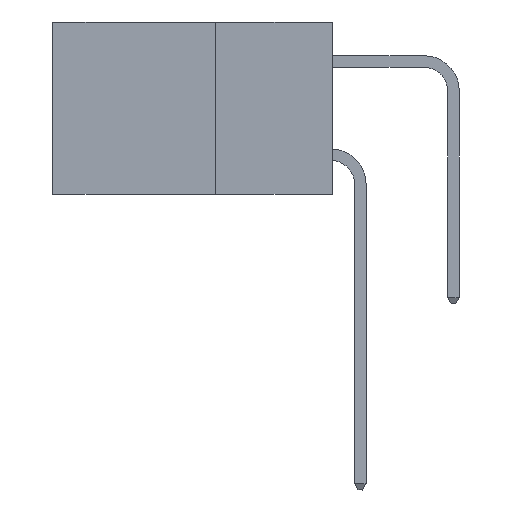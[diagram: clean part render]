
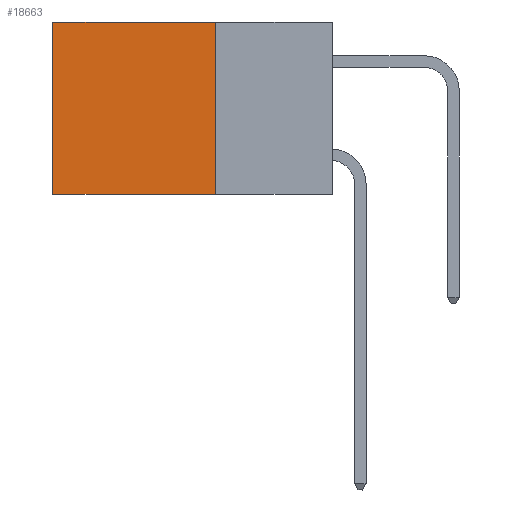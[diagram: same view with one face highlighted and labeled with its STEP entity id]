
A CAD part, left-side view. The second image highlights one B-rep face of the part: STEP entity #18663.
In plain terms, the highlighted planar face has unit normal (-1, 0, 0).
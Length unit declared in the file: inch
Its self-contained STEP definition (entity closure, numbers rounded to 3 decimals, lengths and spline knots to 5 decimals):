
#1170 = ORIENTED_EDGE ( 'NONE', *, *, #32730, .T. ) ;
#2419 = ORIENTED_EDGE ( 'NONE', *, *, #30927, .F. ) ;
#2543 = VERTEX_POINT ( 'NONE', #30915 ) ;
#3652 = EDGE_CURVE ( 'NONE', #2543, #19831, #21561, .T. ) ;
#4007 = DIRECTION ( 'NONE',  ( 0., 0., -1. ) ) ;
#4159 = ORIENTED_EDGE ( 'NONE', *, *, #18547, .F. ) ;
#5460 = DIRECTION ( 'NONE',  ( 0., 0., -1. ) ) ;
#5911 = CARTESIAN_POINT ( 'NONE',  ( 0.298, 0.25, 0. ) ) ;
#6156 = VERTEX_POINT ( 'NONE', #27625 ) ;
#9090 = CARTESIAN_POINT ( 'NONE',  ( 0.298, 0.6, 0. ) ) ;
#9427 = DIRECTION ( 'NONE',  ( 0., 1., 0. ) ) ;
#9645 = VECTOR ( 'NONE', #29064, 39.37008 ) ;
#11065 = DIRECTION ( 'NONE',  ( 1., 0., 0. ) ) ;
#11701 = VECTOR ( 'NONE', #9427, 39.37008 ) ;
#12556 = CARTESIAN_POINT ( 'NONE',  ( 0.298, 0.6, 0. ) ) ;
#18429 = VERTEX_POINT ( 'NONE', #20338 ) ;
#18547 = EDGE_CURVE ( 'NONE', #2543, #6156, #22282, .T. ) ;
#18663 = ADVANCED_FACE ( 'NONE', ( #32975 ), #26334, .F. ) ;
#19831 = VERTEX_POINT ( 'NONE', #12556 ) ;
#20338 = CARTESIAN_POINT ( 'NONE',  ( 0.298, 0.6, -0.37 ) ) ;
#20563 = ORIENTED_EDGE ( 'NONE', *, *, #3652, .T. ) ;
#21476 = VECTOR ( 'NONE', #5460, 39.37008 ) ;
#21561 = LINE ( 'NONE', #29028, #9645 ) ;
#21994 = AXIS2_PLACEMENT_3D ( 'NONE', #5911, #11065, #28898 ) ;
#22282 = LINE ( 'NONE', #23331, #21476 ) ;
#23331 = CARTESIAN_POINT ( 'NONE',  ( 0.298, 0.25, 0. ) ) ;
#23530 = VECTOR ( 'NONE', #4007, 39.37008 ) ;
#24338 = LINE ( 'NONE', #9090, #23530 ) ;
#24686 = CARTESIAN_POINT ( 'NONE',  ( 0.298, 0.25, -0.37 ) ) ;
#26334 = PLANE ( 'NONE',  #21994 ) ;
#27625 = CARTESIAN_POINT ( 'NONE',  ( 0.298, 0.25, -0.37 ) ) ;
#27680 = EDGE_LOOP ( 'NONE', ( #1170, #2419, #4159, #20563 ) ) ;
#28898 = DIRECTION ( 'NONE',  ( 0., 0., -1. ) ) ;
#29028 = CARTESIAN_POINT ( 'NONE',  ( 0.298, 0.25, 0. ) ) ;
#29064 = DIRECTION ( 'NONE',  ( 0., 1., 0. ) ) ;
#30915 = CARTESIAN_POINT ( 'NONE',  ( 0.298, 0.25, 0. ) ) ;
#30927 = EDGE_CURVE ( 'NONE', #6156, #18429, #32001, .T. ) ;
#32001 = LINE ( 'NONE', #24686, #11701 ) ;
#32730 = EDGE_CURVE ( 'NONE', #19831, #18429, #24338, .T. ) ;
#32975 = FACE_OUTER_BOUND ( 'NONE', #27680, .T. ) ;
